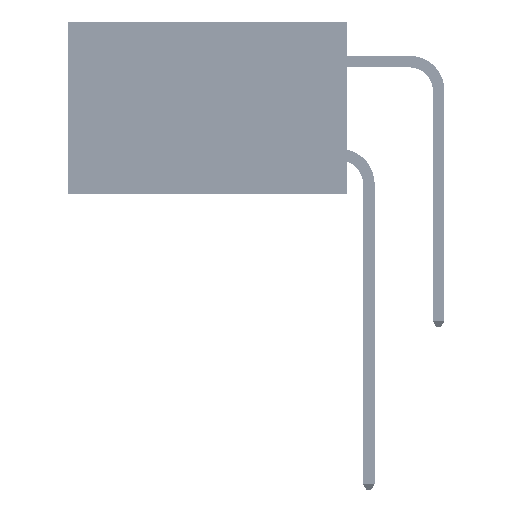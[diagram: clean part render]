
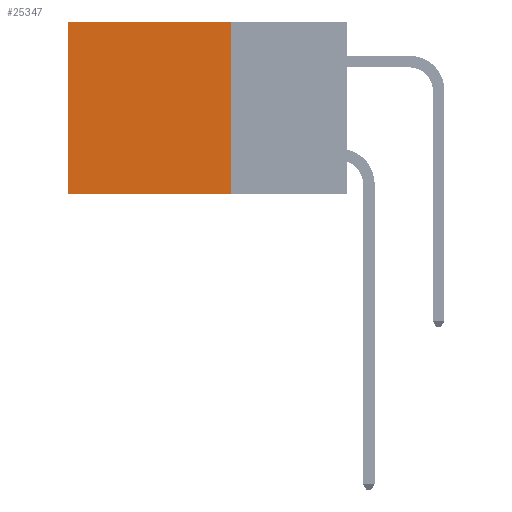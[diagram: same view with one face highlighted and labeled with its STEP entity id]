
A CAD part, left-side view. The second image highlights one B-rep face of the part: STEP entity #25347.
In plain terms, the highlighted planar face has unit normal (-1, 0, 0).
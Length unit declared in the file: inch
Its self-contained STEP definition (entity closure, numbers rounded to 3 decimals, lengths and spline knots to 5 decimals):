
#1572 = VECTOR ( 'NONE', #46833, 39.37008 ) ;
#3021 = VERTEX_POINT ( 'NONE', #35126 ) ;
#3289 = ORIENTED_EDGE ( 'NONE', *, *, #13310, .F. ) ;
#4539 = CARTESIAN_POINT ( 'NONE',  ( 0.2875, 0.25, -0.37 ) ) ;
#6159 = LINE ( 'NONE', #16938, #34246 ) ;
#11694 = VERTEX_POINT ( 'NONE', #33943 ) ;
#12528 = VERTEX_POINT ( 'NONE', #23477 ) ;
#13310 = EDGE_CURVE ( 'NONE', #27317, #12528, #15290, .T. ) ;
#14592 = PLANE ( 'NONE',  #20762 ) ;
#15290 = LINE ( 'NONE', #4539, #1572 ) ;
#16938 = CARTESIAN_POINT ( 'NONE',  ( 0.2875, 0.6, 0. ) ) ;
#17872 = EDGE_CURVE ( 'NONE', #3021, #12528, #6159, .T. ) ;
#18191 = EDGE_LOOP ( 'NONE', ( #33310, #3289, #23655, #28204 ) ) ;
#18242 = DIRECTION ( 'NONE',  ( 0., 0., -1. ) ) ;
#20762 = AXIS2_PLACEMENT_3D ( 'NONE', #29463, #29632, #18242 ) ;
#23477 = CARTESIAN_POINT ( 'NONE',  ( 0.2875, 0.6, -0.37 ) ) ;
#23655 = ORIENTED_EDGE ( 'NONE', *, *, #27618, .F. ) ;
#25347 = ADVANCED_FACE ( 'NONE', ( #39047 ), #14592, .F. ) ;
#25645 = DIRECTION ( 'NONE',  ( 0., 1., 0. ) ) ;
#27317 = VERTEX_POINT ( 'NONE', #46406 ) ;
#27618 = EDGE_CURVE ( 'NONE', #11694, #27317, #43078, .T. ) ;
#28204 = ORIENTED_EDGE ( 'NONE', *, *, #32614, .T. ) ;
#29463 = CARTESIAN_POINT ( 'NONE',  ( 0.2875, 0.25, 0. ) ) ;
#29632 = DIRECTION ( 'NONE',  ( 1., 0., 0. ) ) ;
#32614 = EDGE_CURVE ( 'NONE', #11694, #3021, #33203, .T. ) ;
#33203 = LINE ( 'NONE', #48558, #37419 ) ;
#33310 = ORIENTED_EDGE ( 'NONE', *, *, #17872, .T. ) ;
#33943 = CARTESIAN_POINT ( 'NONE',  ( 0.2875, 0.25, 0. ) ) ;
#34246 = VECTOR ( 'NONE', #47689, 39.37008 ) ;
#35126 = CARTESIAN_POINT ( 'NONE',  ( 0.2875, 0.6, 0. ) ) ;
#36537 = DIRECTION ( 'NONE',  ( 0., 0., -1. ) ) ;
#37419 = VECTOR ( 'NONE', #25645, 39.37008 ) ;
#39047 = FACE_OUTER_BOUND ( 'NONE', #18191, .T. ) ;
#40117 = VECTOR ( 'NONE', #36537, 39.37008 ) ;
#40209 = CARTESIAN_POINT ( 'NONE',  ( 0.2875, 0.25, 0. ) ) ;
#43078 = LINE ( 'NONE', #40209, #40117 ) ;
#46406 = CARTESIAN_POINT ( 'NONE',  ( 0.2875, 0.25, -0.37 ) ) ;
#46833 = DIRECTION ( 'NONE',  ( 0., 1., 0. ) ) ;
#47689 = DIRECTION ( 'NONE',  ( 0., 0., -1. ) ) ;
#48558 = CARTESIAN_POINT ( 'NONE',  ( 0.2875, 0.25, 0. ) ) ;
